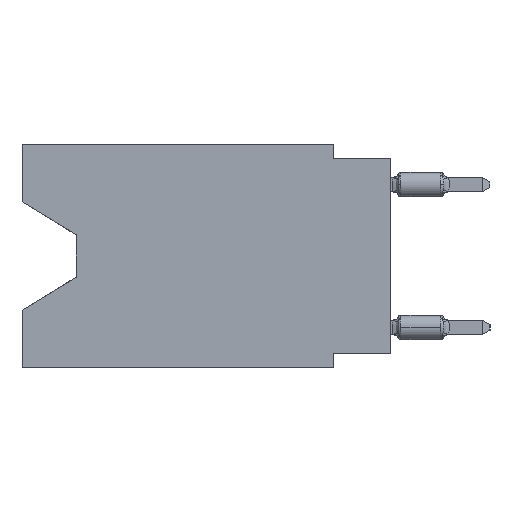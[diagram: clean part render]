
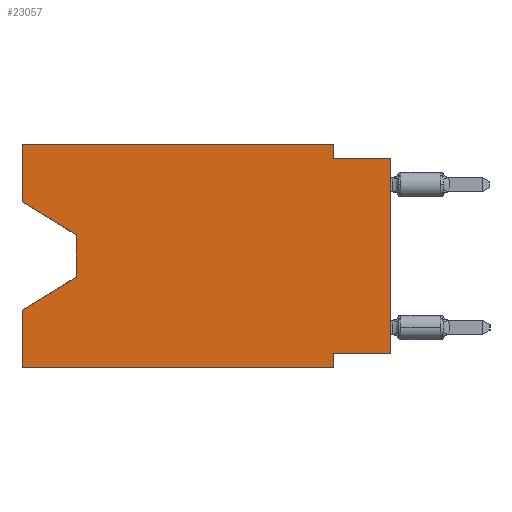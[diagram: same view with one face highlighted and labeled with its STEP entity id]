
A CAD part, left-side view. The second image highlights one B-rep face of the part: STEP entity #23057.
In plain terms, the highlighted planar face has unit normal (-1, 0, 0).
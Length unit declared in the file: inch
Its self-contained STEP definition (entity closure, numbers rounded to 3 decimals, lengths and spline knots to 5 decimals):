
#27 = VERTEX_POINT ( 'NONE', #14462 ) ;
#365 = LINE ( 'NONE', #4179, #23776 ) ;
#519 = CARTESIAN_POINT ( 'NONE',  ( 0., 0.1, -0.39 ) ) ;
#597 = CARTESIAN_POINT ( 'NONE',  ( 0., 0.645, -0.10025 ) ) ;
#718 = LINE ( 'NONE', #4535, #3605 ) ;
#809 = DIRECTION ( 'NONE',  ( 0., 0., -1. ) ) ;
#1051 = VECTOR ( 'NONE', #10677, 39.37008 ) ;
#1396 = VERTEX_POINT ( 'NONE', #519 ) ;
#2206 = VECTOR ( 'NONE', #16719, 39.37008 ) ;
#2461 = DIRECTION ( 'NONE',  ( 0., 0., 1. ) ) ;
#2511 = VERTEX_POINT ( 'NONE', #5999 ) ;
#2838 = DIRECTION ( 'NONE',  ( 0., 0., 1. ) ) ;
#2897 = VERTEX_POINT ( 'NONE', #9057 ) ;
#3452 = DIRECTION ( 'NONE',  ( 0., 0., 1. ) ) ;
#3605 = VECTOR ( 'NONE', #11819, 39.37008 ) ;
#3887 = CARTESIAN_POINT ( 'NONE',  ( 0., 0.645, 0. ) ) ;
#4024 = VERTEX_POINT ( 'NONE', #23407 ) ;
#4179 = CARTESIAN_POINT ( 'NONE',  ( 0., 0.1, 0. ) ) ;
#4254 = VERTEX_POINT ( 'NONE', #16975 ) ;
#4535 = CARTESIAN_POINT ( 'NONE',  ( 0., 0., -0.025 ) ) ;
#4817 = EDGE_CURVE ( 'NONE', #24166, #2511, #24170, .T. ) ;
#4911 = CARTESIAN_POINT ( 'NONE',  ( 0., 0.1, -0.39 ) ) ;
#5389 = VECTOR ( 'NONE', #20283, 39.37008 ) ;
#5421 = LINE ( 'NONE', #12940, #11147 ) ;
#5481 = EDGE_LOOP ( 'NONE', ( #8758, #9731, #15566, #6637, #16568, #12617, #10208, #10939, #13292, #10817, #8823, #13203 ) ) ;
#5865 = VERTEX_POINT ( 'NONE', #18523 ) ;
#5999 = CARTESIAN_POINT ( 'NONE',  ( 0., 0.1, -0.365 ) ) ;
#6043 = EDGE_CURVE ( 'NONE', #2897, #19691, #718, .T. ) ;
#6221 = CARTESIAN_POINT ( 'NONE',  ( 0., 0.645, 0. ) ) ;
#6637 = ORIENTED_EDGE ( 'NONE', *, *, #7690, .F. ) ;
#6710 = CARTESIAN_POINT ( 'NONE',  ( 0., 0.55, -0.158 ) ) ;
#7581 = CARTESIAN_POINT ( 'NONE',  ( 0., 0.55, -0.232 ) ) ;
#7690 = EDGE_CURVE ( 'NONE', #4024, #5865, #8245, .T. ) ;
#7817 = DIRECTION ( 'NONE',  ( 0., -1., 0. ) ) ;
#8081 = EDGE_CURVE ( 'NONE', #4254, #17602, #15223, .T. ) ;
#8182 = CARTESIAN_POINT ( 'NONE',  ( 0., 0.1, 0. ) ) ;
#8245 = LINE ( 'NONE', #15767, #11097 ) ;
#8568 = LINE ( 'NONE', #22023, #1051 ) ;
#8758 = ORIENTED_EDGE ( 'NONE', *, *, #22915, .T. ) ;
#8823 = ORIENTED_EDGE ( 'NONE', *, *, #8081, .F. ) ;
#8950 = EDGE_CURVE ( 'NONE', #17602, #2897, #365, .T. ) ;
#9057 = CARTESIAN_POINT ( 'NONE',  ( 0., 0.1, -0.025 ) ) ;
#9082 = EDGE_CURVE ( 'NONE', #2511, #1396, #16003, .T. ) ;
#9731 = ORIENTED_EDGE ( 'NONE', *, *, #10056, .T. ) ;
#10056 = EDGE_CURVE ( 'NONE', #21331, #27, #14121, .T. ) ;
#10208 = ORIENTED_EDGE ( 'NONE', *, *, #4817, .F. ) ;
#10677 = DIRECTION ( 'NONE',  ( 0., -0.855, -0.519 ) ) ;
#10817 = ORIENTED_EDGE ( 'NONE', *, *, #8950, .F. ) ;
#10939 = ORIENTED_EDGE ( 'NONE', *, *, #15383, .T. ) ;
#11094 = VECTOR ( 'NONE', #2838, 39.37008 ) ;
#11097 = VECTOR ( 'NONE', #2461, 39.37008 ) ;
#11147 = VECTOR ( 'NONE', #3452, 39.37008 ) ;
#11819 = DIRECTION ( 'NONE',  ( 0., -1., 0. ) ) ;
#12049 = CARTESIAN_POINT ( 'NONE',  ( 0., 0., -0.025 ) ) ;
#12151 = CARTESIAN_POINT ( 'NONE',  ( 0., 0.55, -0.158 ) ) ;
#12270 = VECTOR ( 'NONE', #7817, 39.37008 ) ;
#12617 = ORIENTED_EDGE ( 'NONE', *, *, #9082, .F. ) ;
#12940 = CARTESIAN_POINT ( 'NONE',  ( 0., 0., 0. ) ) ;
#13143 = LINE ( 'NONE', #7581, #2206 ) ;
#13203 = ORIENTED_EDGE ( 'NONE', *, *, #13981, .F. ) ;
#13292 = ORIENTED_EDGE ( 'NONE', *, *, #6043, .F. ) ;
#13981 = EDGE_CURVE ( 'NONE', #22343, #4254, #19841, .T. ) ;
#14121 = LINE ( 'NONE', #6710, #15555 ) ;
#14462 = CARTESIAN_POINT ( 'NONE',  ( 0., 0.55, -0.232 ) ) ;
#14922 = CARTESIAN_POINT ( 'NONE',  ( 0., 0., -0.365 ) ) ;
#15223 = LINE ( 'NONE', #6221, #12270 ) ;
#15346 = FACE_OUTER_BOUND ( 'NONE', #5481, .T. ) ;
#15383 = EDGE_CURVE ( 'NONE', #24166, #19691, #5421, .T. ) ;
#15555 = VECTOR ( 'NONE', #809, 39.37008 ) ;
#15566 = ORIENTED_EDGE ( 'NONE', *, *, #19907, .T. ) ;
#15585 = PLANE ( 'NONE',  #20741 ) ;
#15651 = DIRECTION ( 'NONE',  ( 0., 0., -1. ) ) ;
#15767 = CARTESIAN_POINT ( 'NONE',  ( 0., 0.645, 0. ) ) ;
#16003 = LINE ( 'NONE', #4911, #23395 ) ;
#16568 = ORIENTED_EDGE ( 'NONE', *, *, #22929, .T. ) ;
#16719 = DIRECTION ( 'NONE',  ( 0., 0.855, -0.519 ) ) ;
#16953 = LINE ( 'NONE', #23996, #5389 ) ;
#16975 = CARTESIAN_POINT ( 'NONE',  ( 0., 0.645, 0. ) ) ;
#17602 = VERTEX_POINT ( 'NONE', #8182 ) ;
#17699 = CARTESIAN_POINT ( 'NONE',  ( 0., 0., -0.365 ) ) ;
#18523 = CARTESIAN_POINT ( 'NONE',  ( 0., 0.645, -0.28975 ) ) ;
#18926 = DIRECTION ( 'NONE',  ( 0., 0., -1. ) ) ;
#19293 = DIRECTION ( 'NONE',  ( 1., 0., 0. ) ) ;
#19691 = VERTEX_POINT ( 'NONE', #12049 ) ;
#19841 = LINE ( 'NONE', #21817, #11094 ) ;
#19907 = EDGE_CURVE ( 'NONE', #27, #5865, #13143, .T. ) ;
#20283 = DIRECTION ( 'NONE',  ( 0., -1., 0. ) ) ;
#20741 = AXIS2_PLACEMENT_3D ( 'NONE', #3887, #19293, #18926 ) ;
#21293 = VECTOR ( 'NONE', #23802, 39.37008 ) ;
#21331 = VERTEX_POINT ( 'NONE', #12151 ) ;
#21817 = CARTESIAN_POINT ( 'NONE',  ( 0., 0.645, 0. ) ) ;
#22023 = CARTESIAN_POINT ( 'NONE',  ( 0., 0.645, -0.10025 ) ) ;
#22343 = VERTEX_POINT ( 'NONE', #597 ) ;
#22683 = DIRECTION ( 'NONE',  ( 0., 0., -1. ) ) ;
#22915 = EDGE_CURVE ( 'NONE', #22343, #21331, #8568, .T. ) ;
#22929 = EDGE_CURVE ( 'NONE', #4024, #1396, #16953, .T. ) ;
#23057 = ADVANCED_FACE ( 'NONE', ( #15346 ), #15585, .F. ) ;
#23395 = VECTOR ( 'NONE', #15651, 39.37008 ) ;
#23407 = CARTESIAN_POINT ( 'NONE',  ( 0., 0.645, -0.39 ) ) ;
#23776 = VECTOR ( 'NONE', #22683, 39.37008 ) ;
#23802 = DIRECTION ( 'NONE',  ( 0., 1., 0. ) ) ;
#23996 = CARTESIAN_POINT ( 'NONE',  ( 0., 0.645, -0.39 ) ) ;
#24166 = VERTEX_POINT ( 'NONE', #17699 ) ;
#24170 = LINE ( 'NONE', #14922, #21293 ) ;
